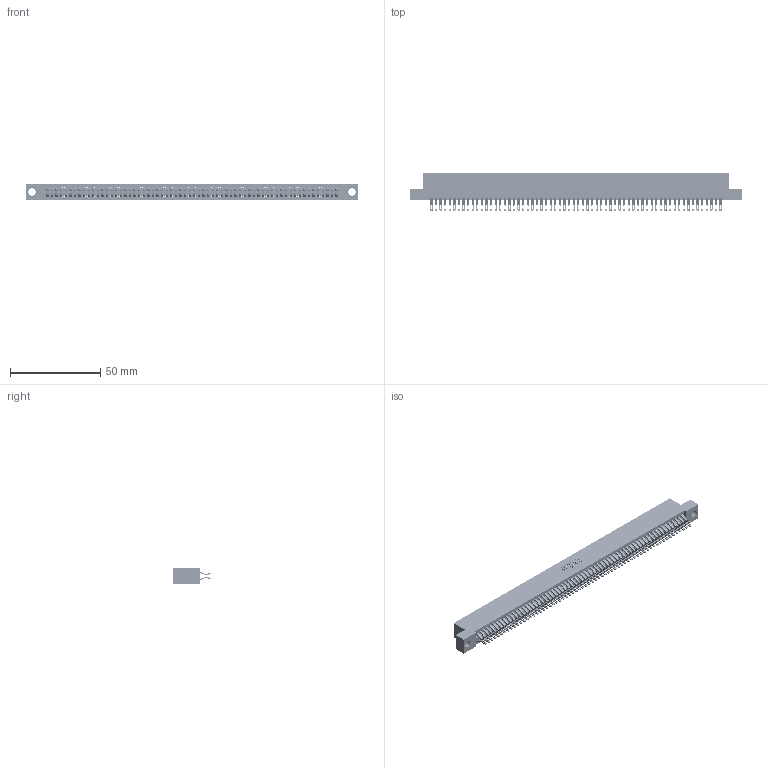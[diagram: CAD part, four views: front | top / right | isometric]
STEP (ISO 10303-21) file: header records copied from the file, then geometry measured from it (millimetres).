
FILE_DESCRIPTION (( 'STEP AP203' ), '1' );
FILE_NAME ('395-128-555-204.STEP', '2018-12-04T12:37:48', ( '' ), ( '' ), 'SwSTEP 2.0', 'SolidWorks 2016', '' );
FILE_SCHEMA (( 'CONFIG_CONTROL_DESIGN' ));
Length unit declared in the file: inch
Products named in the file (3): 345-292-001_555 Tail; 395-128-555-204; 345 Part_Flush Mounting Lugs - 0.156 Dia-TH
Assembly tree (129 placements, depth 2):
  395-128-555-204
    345 Part_Flush Mounting Lugs - 0.156 Dia-TH
    345-292-001_555 Tail  x128
Bounding box: 183.77 x 21.13 x 9.4 mm (x, y, z)
Volume: 18339.1 mm3; surface area: 28640.9 mm2
Topology: 129 solids, 129 shells, 7294 faces, 22997 edges, 15330 vertices
Faces by surface type: plane 4048, cylinder 3246
Entity records: 47583 total; most frequent: CARTESIAN_POINT 7990, ORIENTED_EDGE 7894, DIRECTION 6987, EDGE_CURVE 3947, LINE 3539, VECTOR 3539, VERTEX_POINT 2630, AXIS2_PLACEMENT_3D 1724
